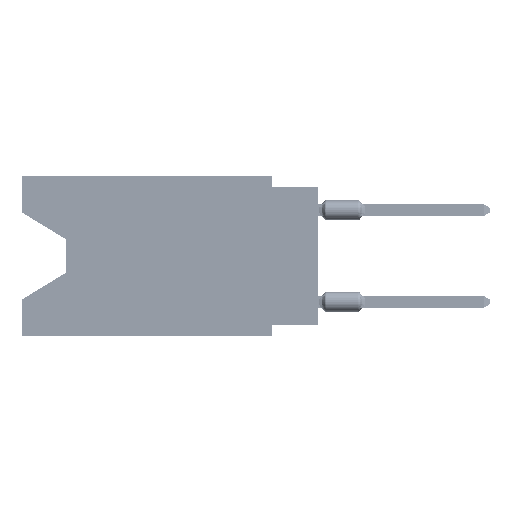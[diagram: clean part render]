
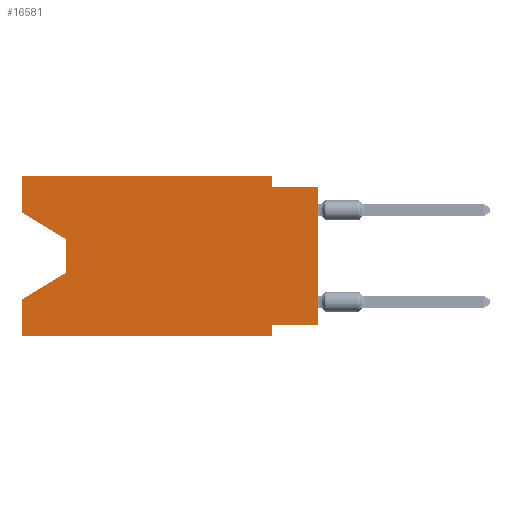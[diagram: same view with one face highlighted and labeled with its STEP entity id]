
A CAD part, left-side view. The second image highlights one B-rep face of the part: STEP entity #16581.
In plain terms, the highlighted planar face has unit normal (-1, 0, 0).
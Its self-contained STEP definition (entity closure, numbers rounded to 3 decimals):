
#977 = LINE ( 'NONE', #69081, #63498 ) ;
#1184 = DIRECTION ( 'NONE',  ( 1., 0., 0. ) ) ;
#2646 = LINE ( 'NONE', #19577, #52849 ) ;
#2842 = LINE ( 'NONE', #35026, #35511 ) ;
#4998 = CARTESIAN_POINT ( 'NONE',  ( 0., 16.383, -2.038 ) ) ;
#6164 = CARTESIAN_POINT ( 'NONE',  ( 0., 16.383, 0. ) ) ;
#6646 = CARTESIAN_POINT ( 'NONE',  ( 0., 2.54, -8.89 ) ) ;
#7398 = LINE ( 'NONE', #33389, #79164 ) ;
#8217 = DIRECTION ( 'NONE',  ( 0., 0., 1. ) ) ;
#8282 = CARTESIAN_POINT ( 'NONE',  ( 0., 0., -0.635 ) ) ;
#8502 = ORIENTED_EDGE ( 'NONE', *, *, #45024, .F. ) ;
#10088 = EDGE_CURVE ( 'NONE', #30054, #41250, #7398, .T. ) ;
#10611 = VECTOR ( 'NONE', #31564, 1000. ) ;
#12176 = LINE ( 'NONE', #55936, #10611 ) ;
#13295 = EDGE_LOOP ( 'NONE', ( #67364, #78638, #41492, #60305, #72168, #36052, #28217, #54335, #74799, #76945, #21326, #8502 ) ) ;
#13327 = CARTESIAN_POINT ( 'NONE',  ( 0., 13.97, -3.505 ) ) ;
#14803 = LINE ( 'NONE', #34190, #67124 ) ;
#16581 = ADVANCED_FACE ( 'NONE', ( #63082 ), #76700, .F. ) ;
#18514 = VECTOR ( 'NONE', #24571, 1000. ) ;
#18937 = DIRECTION ( 'NONE',  ( 0., 0., -1. ) ) ;
#19140 = VERTEX_POINT ( 'NONE', #23720 ) ;
#19577 = CARTESIAN_POINT ( 'NONE',  ( 0., 16.383, -8.89 ) ) ;
#19997 = DIRECTION ( 'NONE',  ( 0., -1., 0. ) ) ;
#21326 = ORIENTED_EDGE ( 'NONE', *, *, #41780, .F. ) ;
#21406 = VECTOR ( 'NONE', #29760, 1000. ) ;
#22661 = VECTOR ( 'NONE', #63951, 1000. ) ;
#23720 = CARTESIAN_POINT ( 'NONE',  ( 0., 0., -8.255 ) ) ;
#23770 = LINE ( 'NONE', #74112, #18514 ) ;
#24571 = DIRECTION ( 'NONE',  ( 0., -1., 0. ) ) ;
#26018 = EDGE_CURVE ( 'NONE', #19140, #36014, #78706, .T. ) ;
#26563 = DIRECTION ( 'NONE',  ( 0., -0.855, -0.519 ) ) ;
#28170 = CARTESIAN_POINT ( 'NONE',  ( 0., 13.97, -5.385 ) ) ;
#28217 = ORIENTED_EDGE ( 'NONE', *, *, #81233, .F. ) ;
#28785 = VERTEX_POINT ( 'NONE', #13327 ) ;
#29760 = DIRECTION ( 'NONE',  ( 0., 0., -1. ) ) ;
#30054 = VERTEX_POINT ( 'NONE', #28170 ) ;
#31564 = DIRECTION ( 'NONE',  ( 0., 1., 0. ) ) ;
#32216 = EDGE_CURVE ( 'NONE', #49533, #36014, #64793, .T. ) ;
#33389 = CARTESIAN_POINT ( 'NONE',  ( 0., 13.97, -5.385 ) ) ;
#33419 = LINE ( 'NONE', #70568, #22661 ) ;
#34190 = CARTESIAN_POINT ( 'NONE',  ( 0., 13.97, -3.505 ) ) ;
#34315 = LINE ( 'NONE', #59483, #21406 ) ;
#34951 = CARTESIAN_POINT ( 'NONE',  ( 0., 2.54, -0.635 ) ) ;
#35026 = CARTESIAN_POINT ( 'NONE',  ( 0., 16.383, 0. ) ) ;
#35511 = VECTOR ( 'NONE', #8217, 1000. ) ;
#35779 = CARTESIAN_POINT ( 'NONE',  ( 0., 16.383, -8.89 ) ) ;
#36014 = VERTEX_POINT ( 'NONE', #70891 ) ;
#36052 = ORIENTED_EDGE ( 'NONE', *, *, #76008, .F. ) ;
#39391 = CARTESIAN_POINT ( 'NONE',  ( 0., 2.54, 0. ) ) ;
#39946 = CARTESIAN_POINT ( 'NONE',  ( 0., 16.383, 0. ) ) ;
#40387 = VECTOR ( 'NONE', #66023, 1000. ) ;
#41250 = VERTEX_POINT ( 'NONE', #63147 ) ;
#41492 = ORIENTED_EDGE ( 'NONE', *, *, #10088, .T. ) ;
#41780 = EDGE_CURVE ( 'NONE', #53805, #72554, #23770, .T. ) ;
#42380 = VECTOR ( 'NONE', #73750, 1000. ) ;
#44546 = VERTEX_POINT ( 'NONE', #35779 ) ;
#45024 = EDGE_CURVE ( 'NONE', #73292, #53805, #33419, .T. ) ;
#45298 = CARTESIAN_POINT ( 'NONE',  ( 0., 2.54, -8.255 ) ) ;
#46998 = DIRECTION ( 'NONE',  ( 0., 0., -1. ) ) ;
#48366 = LINE ( 'NONE', #66929, #51587 ) ;
#49533 = VERTEX_POINT ( 'NONE', #34951 ) ;
#51587 = VECTOR ( 'NONE', #60335, 1000. ) ;
#52587 = EDGE_CURVE ( 'NONE', #28785, #30054, #14803, .T. ) ;
#52594 = EDGE_CURVE ( 'NONE', #44546, #41250, #2842, .T. ) ;
#52849 = VECTOR ( 'NONE', #19997, 1000. ) ;
#53805 = VERTEX_POINT ( 'NONE', #39946 ) ;
#54335 = ORIENTED_EDGE ( 'NONE', *, *, #26018, .T. ) ;
#54431 = VERTEX_POINT ( 'NONE', #6646 ) ;
#55741 = EDGE_CURVE ( 'NONE', #73292, #28785, #977, .T. ) ;
#55936 = CARTESIAN_POINT ( 'NONE',  ( 0., 0., -8.255 ) ) ;
#58029 = EDGE_CURVE ( 'NONE', #72554, #49533, #34315, .T. ) ;
#59483 = CARTESIAN_POINT ( 'NONE',  ( 0., 2.54, 0. ) ) ;
#60305 = ORIENTED_EDGE ( 'NONE', *, *, #52594, .F. ) ;
#60335 = DIRECTION ( 'NONE',  ( 0., 0., -1. ) ) ;
#63082 = FACE_OUTER_BOUND ( 'NONE', #13295, .T. ) ;
#63147 = CARTESIAN_POINT ( 'NONE',  ( 0., 16.383, -6.852 ) ) ;
#63498 = VECTOR ( 'NONE', #26563, 1000. ) ;
#63951 = DIRECTION ( 'NONE',  ( 0., 0., 1. ) ) ;
#64793 = LINE ( 'NONE', #8282, #40387 ) ;
#66023 = DIRECTION ( 'NONE',  ( 0., -1., 0. ) ) ;
#66929 = CARTESIAN_POINT ( 'NONE',  ( 0., 2.54, -8.89 ) ) ;
#67124 = VECTOR ( 'NONE', #46998, 1000. ) ;
#67137 = CARTESIAN_POINT ( 'NONE',  ( 0., 0., 0. ) ) ;
#67364 = ORIENTED_EDGE ( 'NONE', *, *, #55741, .T. ) ;
#69081 = CARTESIAN_POINT ( 'NONE',  ( 0., 16.383, -2.038 ) ) ;
#69314 = DIRECTION ( 'NONE',  ( 0., 0.855, -0.519 ) ) ;
#70568 = CARTESIAN_POINT ( 'NONE',  ( 0., 16.383, 0. ) ) ;
#70891 = CARTESIAN_POINT ( 'NONE',  ( 0., 0., -0.635 ) ) ;
#72168 = ORIENTED_EDGE ( 'NONE', *, *, #81404, .T. ) ;
#72554 = VERTEX_POINT ( 'NONE', #39391 ) ;
#73292 = VERTEX_POINT ( 'NONE', #4998 ) ;
#73750 = DIRECTION ( 'NONE',  ( 0., 0., 1. ) ) ;
#74112 = CARTESIAN_POINT ( 'NONE',  ( 0., 16.383, 0. ) ) ;
#74799 = ORIENTED_EDGE ( 'NONE', *, *, #32216, .F. ) ;
#75071 = VERTEX_POINT ( 'NONE', #45298 ) ;
#76008 = EDGE_CURVE ( 'NONE', #75071, #54431, #48366, .T. ) ;
#76700 = PLANE ( 'NONE',  #78376 ) ;
#76945 = ORIENTED_EDGE ( 'NONE', *, *, #58029, .F. ) ;
#78376 = AXIS2_PLACEMENT_3D ( 'NONE', #6164, #1184, #18937 ) ;
#78638 = ORIENTED_EDGE ( 'NONE', *, *, #52587, .T. ) ;
#78706 = LINE ( 'NONE', #67137, #42380 ) ;
#79164 = VECTOR ( 'NONE', #69314, 1000. ) ;
#81233 = EDGE_CURVE ( 'NONE', #19140, #75071, #12176, .T. ) ;
#81404 = EDGE_CURVE ( 'NONE', #44546, #54431, #2646, .T. ) ;
